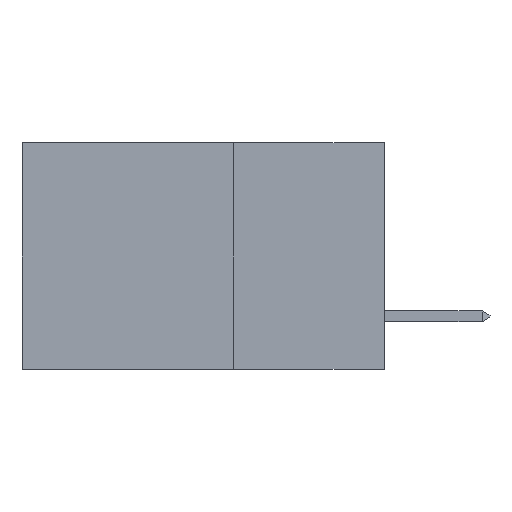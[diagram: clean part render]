
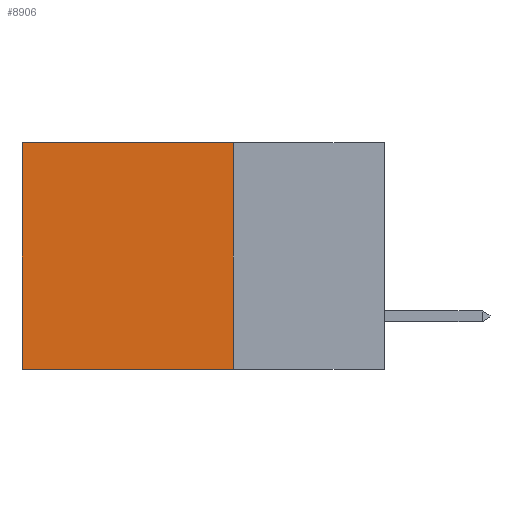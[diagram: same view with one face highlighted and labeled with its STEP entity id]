
A CAD part, left-side view. The second image highlights one B-rep face of the part: STEP entity #8906.
In plain terms, the highlighted planar face has unit normal (-1, 0, 0).
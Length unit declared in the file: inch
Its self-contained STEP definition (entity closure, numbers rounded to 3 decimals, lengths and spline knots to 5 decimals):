
#174 = CARTESIAN_POINT ( 'NONE',  ( 0.2875, 0.6, 0. ) ) ;
#453 = CARTESIAN_POINT ( 'NONE',  ( 0.2875, 0.25, -0.375 ) ) ;
#672 = LINE ( 'NONE', #13023, #2398 ) ;
#787 = EDGE_CURVE ( 'NONE', #8098, #8710, #12978, .T. ) ;
#818 = VERTEX_POINT ( 'NONE', #1957 ) ;
#1134 = EDGE_CURVE ( 'NONE', #10023, #8098, #672, .T. ) ;
#1345 = PLANE ( 'NONE',  #7951 ) ;
#1957 = CARTESIAN_POINT ( 'NONE',  ( 0.2875, 0.25, -0.375 ) ) ;
#2398 = VECTOR ( 'NONE', #12033, 39.37008 ) ;
#2833 = LINE ( 'NONE', #9017, #2981 ) ;
#2981 = VECTOR ( 'NONE', #13109, 39.37008 ) ;
#3022 = EDGE_LOOP ( 'NONE', ( #10449, #5049, #7498, #11056 ) ) ;
#3347 = FACE_OUTER_BOUND ( 'NONE', #3022, .T. ) ;
#4366 = DIRECTION ( 'NONE',  ( 1., 0., 0. ) ) ;
#5049 = ORIENTED_EDGE ( 'NONE', *, *, #10618, .F. ) ;
#7498 = ORIENTED_EDGE ( 'NONE', *, *, #11413, .F. ) ;
#7951 = AXIS2_PLACEMENT_3D ( 'NONE', #8471, #4366, #9745 ) ;
#8017 = CARTESIAN_POINT ( 'NONE',  ( 0.2875, 0.6, -0.375 ) ) ;
#8098 = VERTEX_POINT ( 'NONE', #174 ) ;
#8471 = CARTESIAN_POINT ( 'NONE',  ( 0.2875, 0.25, -0.375 ) ) ;
#8710 = VERTEX_POINT ( 'NONE', #12160 ) ;
#8906 = ADVANCED_FACE ( 'NONE', ( #3347 ), #1345, .F. ) ;
#9017 = CARTESIAN_POINT ( 'NONE',  ( 0.2875, 0.25, -0.375 ) ) ;
#9670 = LINE ( 'NONE', #453, #12625 ) ;
#9745 = DIRECTION ( 'NONE',  ( 0., 0., -1. ) ) ;
#10023 = VERTEX_POINT ( 'NONE', #13051 ) ;
#10449 = ORIENTED_EDGE ( 'NONE', *, *, #787, .T. ) ;
#10618 = EDGE_CURVE ( 'NONE', #818, #8710, #2833, .T. ) ;
#11056 = ORIENTED_EDGE ( 'NONE', *, *, #1134, .T. ) ;
#11225 = VECTOR ( 'NONE', #12109, 39.37008 ) ;
#11413 = EDGE_CURVE ( 'NONE', #10023, #818, #9670, .T. ) ;
#11423 = DIRECTION ( 'NONE',  ( 0., 0., -1. ) ) ;
#12033 = DIRECTION ( 'NONE',  ( 0., 1., 0. ) ) ;
#12109 = DIRECTION ( 'NONE',  ( 0., 0., -1. ) ) ;
#12160 = CARTESIAN_POINT ( 'NONE',  ( 0.2875, 0.6, -0.375 ) ) ;
#12625 = VECTOR ( 'NONE', #11423, 39.37008 ) ;
#12978 = LINE ( 'NONE', #8017, #11225 ) ;
#13023 = CARTESIAN_POINT ( 'NONE',  ( 0.2875, 0.25, 0. ) ) ;
#13051 = CARTESIAN_POINT ( 'NONE',  ( 0.2875, 0.25, 0. ) ) ;
#13109 = DIRECTION ( 'NONE',  ( 0., 1., 0. ) ) ;
